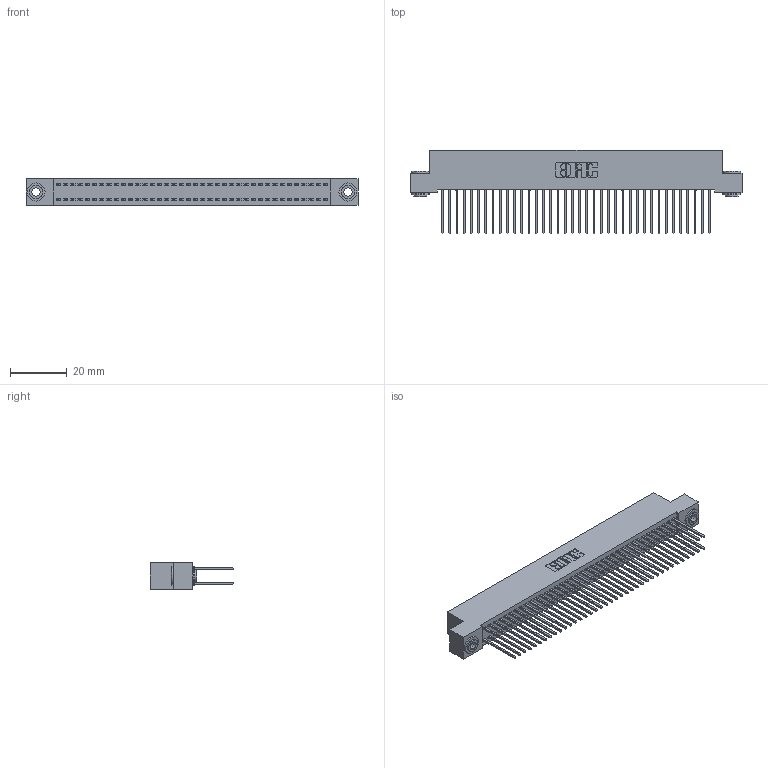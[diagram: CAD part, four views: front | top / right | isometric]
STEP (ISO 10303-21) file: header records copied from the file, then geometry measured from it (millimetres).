
FILE_DESCRIPTION (( 'STEP AP203' ), '1' );
FILE_NAME ('342-076-540-203.STEP', '2019-10-04T10:42:22', ( '' ), ( '' ), 'SwSTEP 2.0', 'SolidWorks 2016', '' );
FILE_SCHEMA (( 'CONFIG_CONTROL_DESIGN' ));
Length unit declared in the file: inch
Products named in the file (4): 342 Part_.156 TH; 345-292-001_345-293-140; 342-250-002_345-250-002-102; 342-076-540-203
Assembly tree (79 placements, depth 2):
  342-076-540-203
    342 Part_.156 TH
    345-292-001_345-293-140  x76
    342-250-002_345-250-002-102  x2
Bounding box: 116.84 x 29.47 x 9.4 mm (x, y, z)
Volume: 10790.1 mm3; surface area: 18959.9 mm2
Topology: 79 solids, 79 shells, 4100 faces, 12155 edges, 7998 vertices
Faces by surface type: plane 2812, cylinder 1280, cone 8
Entity records: 25500 total; most frequent: CARTESIAN_POINT 4205, ORIENTED_EDGE 4134, DIRECTION 3633, EDGE_CURVE 2067, LINE 1915, VECTOR 1915, VERTEX_POINT 1374, AXIS2_PLACEMENT_3D 859
